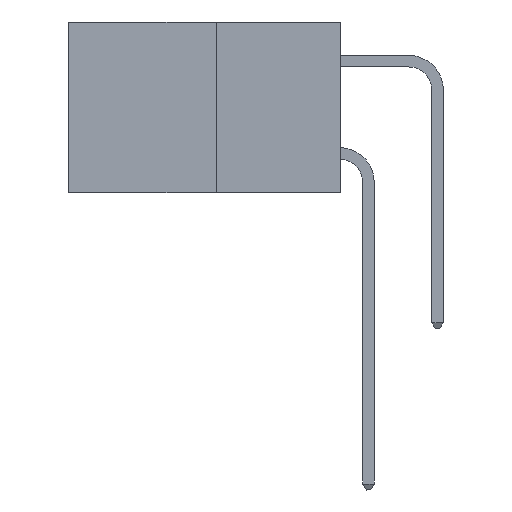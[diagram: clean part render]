
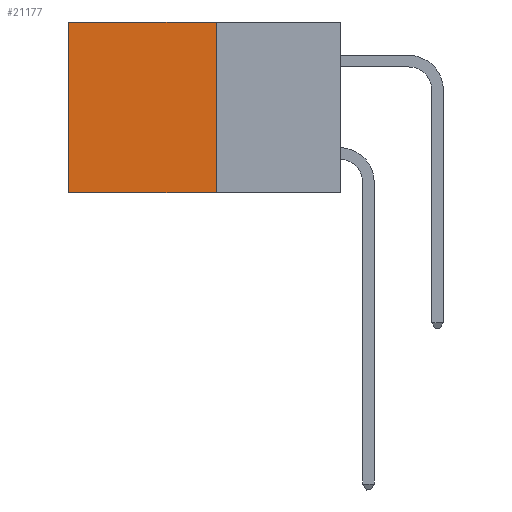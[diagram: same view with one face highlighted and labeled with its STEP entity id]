
A CAD part, left-side view. The second image highlights one B-rep face of the part: STEP entity #21177.
In plain terms, the highlighted planar face has unit normal (-1, 0, 0).
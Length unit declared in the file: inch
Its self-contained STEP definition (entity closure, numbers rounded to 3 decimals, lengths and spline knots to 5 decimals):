
#112 = CARTESIAN_POINT ( 'NONE',  ( 0.277, 0.59, -0.37 ) ) ;
#402 = EDGE_CURVE ( 'NONE', #12079, #1673, #5332, .T. ) ;
#459 = LINE ( 'NONE', #16678, #9575 ) ;
#574 = LINE ( 'NONE', #8006, #4513 ) ;
#752 = EDGE_LOOP ( 'NONE', ( #13494, #11415, #23086, #4626 ) ) ;
#1673 = VERTEX_POINT ( 'NONE', #9835 ) ;
#1856 = DIRECTION ( 'NONE',  ( 1., 0., 0. ) ) ;
#2253 = DIRECTION ( 'NONE',  ( 0., 1., 0. ) ) ;
#2832 = CARTESIAN_POINT ( 'NONE',  ( 0.277, 0.27, -0.37 ) ) ;
#4513 = VECTOR ( 'NONE', #2253, 39.37008 ) ;
#4626 = ORIENTED_EDGE ( 'NONE', *, *, #19495, .T. ) ;
#4713 = VECTOR ( 'NONE', #24705, 39.37008 ) ;
#5332 = LINE ( 'NONE', #112, #4713 ) ;
#7096 = LINE ( 'NONE', #21727, #11643 ) ;
#7179 = VERTEX_POINT ( 'NONE', #7912 ) ;
#7706 = AXIS2_PLACEMENT_3D ( 'NONE', #13436, #1856, #15307 ) ;
#7912 = CARTESIAN_POINT ( 'NONE',  ( 0.277, 0.27, 0. ) ) ;
#7954 = FACE_OUTER_BOUND ( 'NONE', #752, .T. ) ;
#8006 = CARTESIAN_POINT ( 'NONE',  ( 0.277, 0.27, -0.37 ) ) ;
#8892 = EDGE_CURVE ( 'NONE', #7179, #24287, #459, .T. ) ;
#8900 = CARTESIAN_POINT ( 'NONE',  ( 0.277, 0.59, 0. ) ) ;
#9575 = VECTOR ( 'NONE', #18497, 39.37008 ) ;
#9835 = CARTESIAN_POINT ( 'NONE',  ( 0.277, 0.59, -0.37 ) ) ;
#10398 = DIRECTION ( 'NONE',  ( 0., 1., 0. ) ) ;
#11082 = EDGE_CURVE ( 'NONE', #24287, #1673, #574, .T. ) ;
#11415 = ORIENTED_EDGE ( 'NONE', *, *, #11082, .F. ) ;
#11522 = PLANE ( 'NONE',  #7706 ) ;
#11643 = VECTOR ( 'NONE', #10398, 39.37008 ) ;
#12079 = VERTEX_POINT ( 'NONE', #8900 ) ;
#13436 = CARTESIAN_POINT ( 'NONE',  ( 0.277, 0.27, -0.37 ) ) ;
#13494 = ORIENTED_EDGE ( 'NONE', *, *, #402, .T. ) ;
#15307 = DIRECTION ( 'NONE',  ( 0., 0., -1. ) ) ;
#16678 = CARTESIAN_POINT ( 'NONE',  ( 0.277, 0.27, -0.37 ) ) ;
#18497 = DIRECTION ( 'NONE',  ( 0., 0., -1. ) ) ;
#19495 = EDGE_CURVE ( 'NONE', #7179, #12079, #7096, .T. ) ;
#21177 = ADVANCED_FACE ( 'NONE', ( #7954 ), #11522, .F. ) ;
#21727 = CARTESIAN_POINT ( 'NONE',  ( 0.277, 0.27, 0. ) ) ;
#23086 = ORIENTED_EDGE ( 'NONE', *, *, #8892, .F. ) ;
#24287 = VERTEX_POINT ( 'NONE', #2832 ) ;
#24705 = DIRECTION ( 'NONE',  ( 0., 0., -1. ) ) ;
